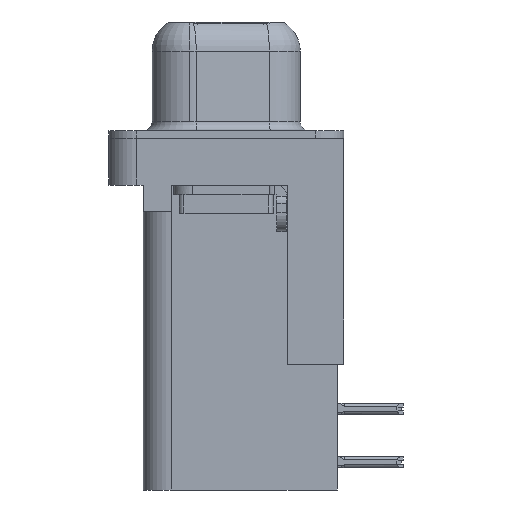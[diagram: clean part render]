
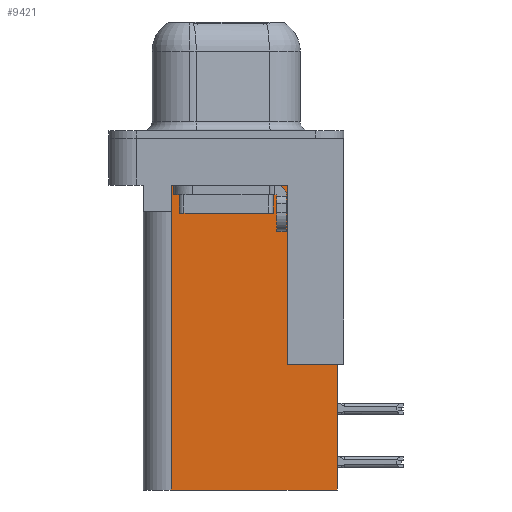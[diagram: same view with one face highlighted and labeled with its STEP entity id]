
A CAD part, left-side view. The second image highlights one B-rep face of the part: STEP entity #9421.
In plain terms, the highlighted planar face has unit normal (-1, 0, 0).
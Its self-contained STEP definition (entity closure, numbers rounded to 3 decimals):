
#79 = DIRECTION ( 'NONE',  ( 0., 1., 0. ) ) ;
#548 = VECTOR ( 'NONE', #12971, 1000. ) ;
#1141 = LINE ( 'NONE', #1907, #548 ) ;
#1907 = CARTESIAN_POINT ( 'NONE',  ( 3.79, 2.895, -3.9 ) ) ;
#1921 = VERTEX_POINT ( 'NONE', #14521 ) ;
#2043 = CARTESIAN_POINT ( 'NONE',  ( 3.79, -3.295, -2.5 ) ) ;
#3182 = LINE ( 'NONE', #9582, #7521 ) ;
#3597 = LINE ( 'NONE', #2043, #9108 ) ;
#4066 = VECTOR ( 'NONE', #19642, 1000. ) ;
#4665 = CARTESIAN_POINT ( 'NONE',  ( 3.79, -5.925, -18.76 ) ) ;
#4675 = VECTOR ( 'NONE', #10415, 1000. ) ;
#4928 = CARTESIAN_POINT ( 'NONE',  ( 3.79, -3.295, -18.76 ) ) ;
#5175 = VECTOR ( 'NONE', #18480, 1000. ) ;
#5312 = ORIENTED_EDGE ( 'NONE', *, *, #19011, .F. ) ;
#5792 = DIRECTION ( 'NONE',  ( 0., 1., 0. ) ) ;
#5977 = DIRECTION ( 'NONE',  ( 0., 1., 0. ) ) ;
#6260 = EDGE_CURVE ( 'NONE', #1921, #22932, #3597, .T. ) ;
#7484 = PLANE ( 'NONE',  #12061 ) ;
#7521 = VECTOR ( 'NONE', #5977, 1000. ) ;
#7629 = EDGE_LOOP ( 'NONE', ( #15903, #11180, #8870, #14221, #18865, #5312, #9074, #22677 ) ) ;
#7983 = VECTOR ( 'NONE', #10102, 1000. ) ;
#8153 = VERTEX_POINT ( 'NONE', #4665 ) ;
#8242 = CARTESIAN_POINT ( 'NONE',  ( 3.79, -5.925, -2. ) ) ;
#8870 = ORIENTED_EDGE ( 'NONE', *, *, #23232, .T. ) ;
#9074 = ORIENTED_EDGE ( 'NONE', *, *, #17352, .T. ) ;
#9108 = VECTOR ( 'NONE', #5792, 1000. ) ;
#9334 = CARTESIAN_POINT ( 'NONE',  ( 3.79, -3.295, -18.76 ) ) ;
#9421 = ADVANCED_FACE ( 'NONE', ( #11326 ), #7484, .F. ) ;
#9561 = LINE ( 'NONE', #4928, #4066 ) ;
#9582 = CARTESIAN_POINT ( 'NONE',  ( 3.79, -3.295, -18.76 ) ) ;
#9591 = LINE ( 'NONE', #23254, #4675 ) ;
#10022 = CARTESIAN_POINT ( 'NONE',  ( 3.79, -5.925, -12.05 ) ) ;
#10077 = LINE ( 'NONE', #22209, #5175 ) ;
#10102 = DIRECTION ( 'NONE',  ( 0., 0., -1. ) ) ;
#10415 = DIRECTION ( 'NONE',  ( 0., 0., 1. ) ) ;
#10528 = VERTEX_POINT ( 'NONE', #23144 ) ;
#11180 = ORIENTED_EDGE ( 'NONE', *, *, #15780, .T. ) ;
#11198 = DIRECTION ( 'NONE',  ( 1., 0., 0. ) ) ;
#11326 = FACE_OUTER_BOUND ( 'NONE', #7629, .T. ) ;
#11364 = VERTEX_POINT ( 'NONE', #10022 ) ;
#12027 = CARTESIAN_POINT ( 'NONE',  ( 3.79, 2.925, -18.76 ) ) ;
#12061 = AXIS2_PLACEMENT_3D ( 'NONE', #9334, #11198, #79 ) ;
#12971 = DIRECTION ( 'NONE',  ( 0., 0., -1. ) ) ;
#13806 = CARTESIAN_POINT ( 'NONE',  ( 3.79, 2.925, -3.9 ) ) ;
#14186 = VECTOR ( 'NONE', #15286, 1000. ) ;
#14221 = ORIENTED_EDGE ( 'NONE', *, *, #22942, .F. ) ;
#14521 = CARTESIAN_POINT ( 'NONE',  ( 3.79, -3.295, -2.5 ) ) ;
#14748 = LINE ( 'NONE', #18896, #14186 ) ;
#15286 = DIRECTION ( 'NONE',  ( 0., 1., 0. ) ) ;
#15537 = EDGE_CURVE ( 'NONE', #16640, #1921, #9561, .T. ) ;
#15780 = EDGE_CURVE ( 'NONE', #22932, #10528, #1141, .T. ) ;
#15903 = ORIENTED_EDGE ( 'NONE', *, *, #6260, .T. ) ;
#15923 = EDGE_CURVE ( 'NONE', #8153, #22852, #3182, .T. ) ;
#15944 = CARTESIAN_POINT ( 'NONE',  ( 3.79, 2.895, -2.5 ) ) ;
#16640 = VERTEX_POINT ( 'NONE', #19097 ) ;
#17352 = EDGE_CURVE ( 'NONE', #11364, #16640, #10077, .T. ) ;
#18480 = DIRECTION ( 'NONE',  ( 0., 1., 0. ) ) ;
#18865 = ORIENTED_EDGE ( 'NONE', *, *, #15923, .F. ) ;
#18896 = CARTESIAN_POINT ( 'NONE',  ( 3.79, 0., -3.9 ) ) ;
#19011 = EDGE_CURVE ( 'NONE', #11364, #8153, #22660, .T. ) ;
#19097 = CARTESIAN_POINT ( 'NONE',  ( 3.79, -3.295, -12.05 ) ) ;
#19642 = DIRECTION ( 'NONE',  ( 0., 0., 1. ) ) ;
#19756 = VERTEX_POINT ( 'NONE', #13806 ) ;
#22209 = CARTESIAN_POINT ( 'NONE',  ( 3.79, -6.295, -12.05 ) ) ;
#22660 = LINE ( 'NONE', #8242, #7983 ) ;
#22677 = ORIENTED_EDGE ( 'NONE', *, *, #15537, .T. ) ;
#22852 = VERTEX_POINT ( 'NONE', #12027 ) ;
#22932 = VERTEX_POINT ( 'NONE', #15944 ) ;
#22942 = EDGE_CURVE ( 'NONE', #22852, #19756, #9591, .T. ) ;
#23144 = CARTESIAN_POINT ( 'NONE',  ( 3.79, 2.895, -3.9 ) ) ;
#23232 = EDGE_CURVE ( 'NONE', #10528, #19756, #14748, .T. ) ;
#23254 = CARTESIAN_POINT ( 'NONE',  ( 3.79, 2.925, -18.76 ) ) ;
